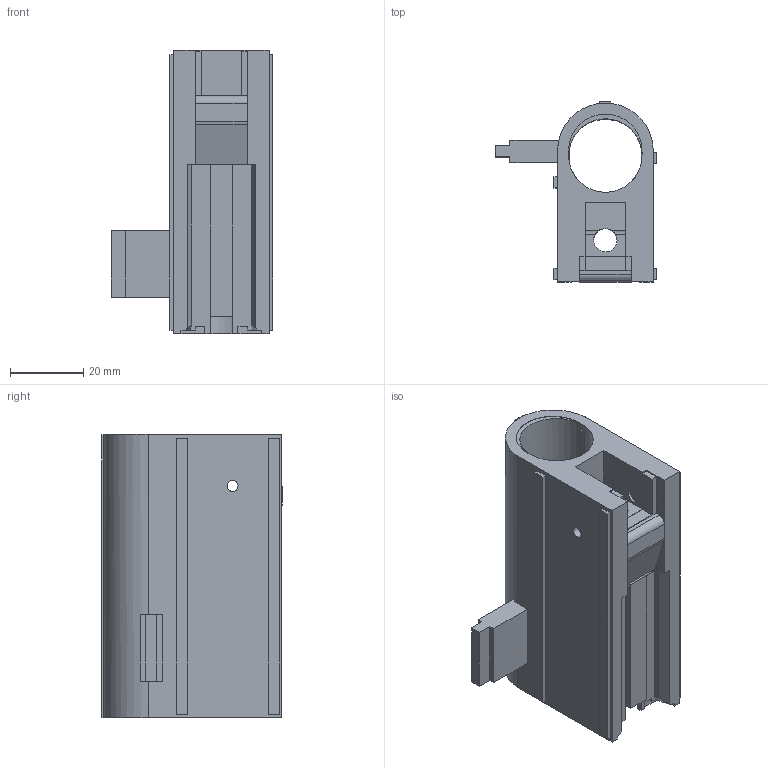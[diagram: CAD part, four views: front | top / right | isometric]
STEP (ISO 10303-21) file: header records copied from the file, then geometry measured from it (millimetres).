
FILE_DESCRIPTION (( 'STEP AP203' ), '1' );
FILE_NAME ('WTF-9MV_bolt_housing.STEP', '2020-05-19T19:42:19', ( '' ), ( '' ), 'SwSTEP 2.0', 'SolidWorks 2016', '' );
FILE_SCHEMA (( 'CONFIG_CONTROL_DESIGN' ));
Length unit declared in the file: millimetre
Products named in the file (1): WTF-9MV_bolt_housing
Bounding box: 44 x 49.1 x 77.19 mm (x, y, z)
Volume: 45394.4 mm3; surface area: 22350.6 mm2
Topology: 1 solids, 3 shells, 163 faces, 454 edges, 301 vertices
Faces by surface type: plane 146, cylinder 17
Full cylindrical faces by diameter (mm): 2.968 x2, 3 x1, 3.566 x1, 6.34 x1, 20 x1
Entity records: 5276 total; most frequent: CARTESIAN_POINT 1009, ORIENTED_EDGE 892, DIRECTION 815, EDGE_CURVE 446, LINE 385, VECTOR 385, VERTEX_POINT 299, AXIS2_PLACEMENT_3D 215
